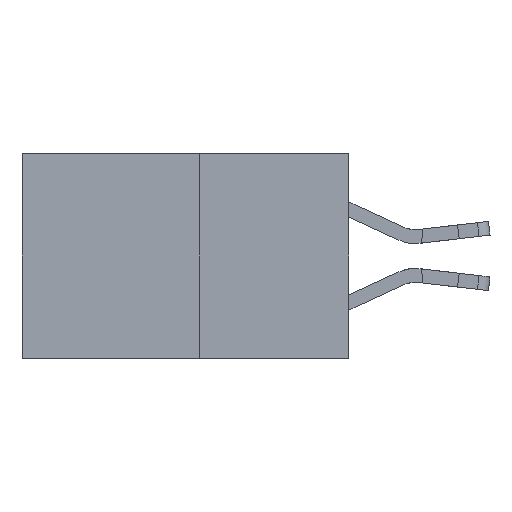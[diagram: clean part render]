
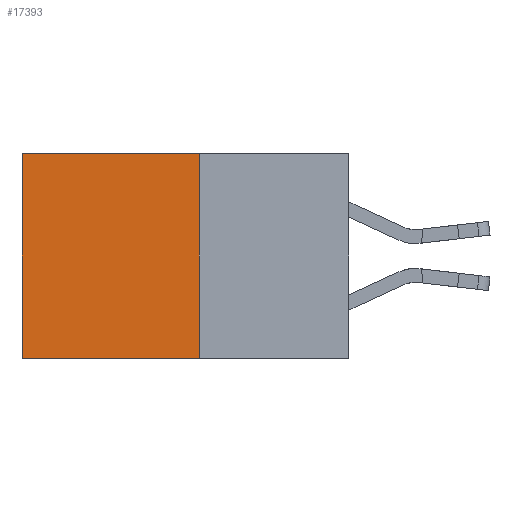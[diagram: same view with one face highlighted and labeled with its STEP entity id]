
A CAD part, left-side view. The second image highlights one B-rep face of the part: STEP entity #17393.
In plain terms, the highlighted planar face has unit normal (-1, 0, 0).
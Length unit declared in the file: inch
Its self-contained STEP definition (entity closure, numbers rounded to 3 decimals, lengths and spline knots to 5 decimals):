
#87 = ORIENTED_EDGE ( 'NONE', *, *, #6723, .F. ) ;
#176 = VERTEX_POINT ( 'NONE', #5256 ) ;
#656 = ORIENTED_EDGE ( 'NONE', *, *, #6853, .F. ) ;
#1041 = ORIENTED_EDGE ( 'NONE', *, *, #9038, .T. ) ;
#1103 = EDGE_CURVE ( 'NONE', #176, #7815, #7077, .T. ) ;
#1536 = EDGE_LOOP ( 'NONE', ( #18376, #87, #656, #1041 ) ) ;
#2373 = DIRECTION ( 'NONE',  ( 1., 0., 0. ) ) ;
#2667 = VECTOR ( 'NONE', #18141, 39.37008 ) ;
#3444 = CARTESIAN_POINT ( 'NONE',  ( 0.277, 0.27, 0. ) ) ;
#3791 = VECTOR ( 'NONE', #6184, 39.37008 ) ;
#3848 = CARTESIAN_POINT ( 'NONE',  ( 0.277, 0.59, -0.37 ) ) ;
#3890 = FACE_OUTER_BOUND ( 'NONE', #1536, .T. ) ;
#4547 = CARTESIAN_POINT ( 'NONE',  ( 0.277, 0.27, -0.37 ) ) ;
#5098 = VERTEX_POINT ( 'NONE', #6522 ) ;
#5256 = CARTESIAN_POINT ( 'NONE',  ( 0.277, 0.59, 0. ) ) ;
#6184 = DIRECTION ( 'NONE',  ( 0., 0., -1. ) ) ;
#6442 = DIRECTION ( 'NONE',  ( 0., 0., -1. ) ) ;
#6457 = CARTESIAN_POINT ( 'NONE',  ( 0.277, 0.59, -0.37 ) ) ;
#6522 = CARTESIAN_POINT ( 'NONE',  ( 0.277, 0.27, -0.37 ) ) ;
#6723 = EDGE_CURVE ( 'NONE', #5098, #7815, #7627, .T. ) ;
#6853 = EDGE_CURVE ( 'NONE', #7842, #5098, #11854, .T. ) ;
#7077 = LINE ( 'NONE', #6457, #15113 ) ;
#7093 = CARTESIAN_POINT ( 'NONE',  ( 0.277, 0.27, -0.37 ) ) ;
#7627 = LINE ( 'NONE', #13309, #14738 ) ;
#7815 = VERTEX_POINT ( 'NONE', #3848 ) ;
#7842 = VERTEX_POINT ( 'NONE', #3444 ) ;
#8571 = PLANE ( 'NONE',  #14948 ) ;
#9038 = EDGE_CURVE ( 'NONE', #7842, #176, #10322, .T. ) ;
#10322 = LINE ( 'NONE', #19497, #2667 ) ;
#11854 = LINE ( 'NONE', #4547, #3791 ) ;
#13034 = DIRECTION ( 'NONE',  ( 0., 1., 0. ) ) ;
#13309 = CARTESIAN_POINT ( 'NONE',  ( 0.277, 0.27, -0.37 ) ) ;
#14738 = VECTOR ( 'NONE', #13034, 39.37008 ) ;
#14948 = AXIS2_PLACEMENT_3D ( 'NONE', #7093, #2373, #18977 ) ;
#15113 = VECTOR ( 'NONE', #6442, 39.37008 ) ;
#17393 = ADVANCED_FACE ( 'NONE', ( #3890 ), #8571, .F. ) ;
#18141 = DIRECTION ( 'NONE',  ( 0., 1., 0. ) ) ;
#18376 = ORIENTED_EDGE ( 'NONE', *, *, #1103, .T. ) ;
#18977 = DIRECTION ( 'NONE',  ( 0., 0., -1. ) ) ;
#19497 = CARTESIAN_POINT ( 'NONE',  ( 0.277, 0.27, 0. ) ) ;
